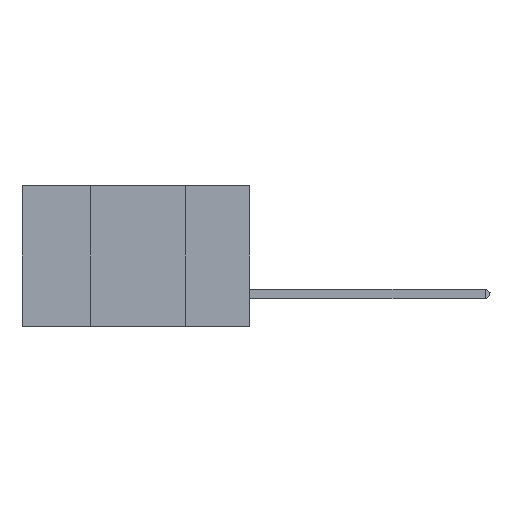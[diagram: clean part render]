
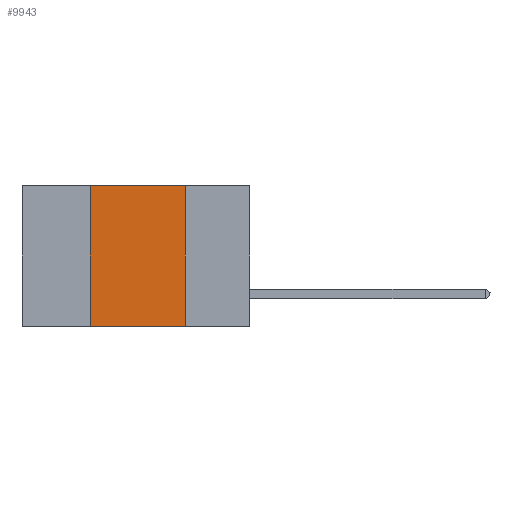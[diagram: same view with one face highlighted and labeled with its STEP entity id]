
A CAD part, left-side view. The second image highlights one B-rep face of the part: STEP entity #9943.
In plain terms, the highlighted planar face has unit normal (-1, 0, 0).
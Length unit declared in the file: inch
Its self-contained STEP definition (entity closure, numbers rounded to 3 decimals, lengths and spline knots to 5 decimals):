
#1324 = DIRECTION ( 'NONE',  ( 0., 0., -1. ) ) ;
#1673 = VERTEX_POINT ( 'NONE', #23737 ) ;
#1791 = VERTEX_POINT ( 'NONE', #7109 ) ;
#2474 = CARTESIAN_POINT ( 'NONE',  ( 0., 0.6, -0.37 ) ) ;
#3134 = EDGE_LOOP ( 'NONE', ( #27689, #11336, #5926, #3174 ) ) ;
#3174 = ORIENTED_EDGE ( 'NONE', *, *, #14783, .T. ) ;
#4747 = DIRECTION ( 'NONE',  ( 0., -1., 0. ) ) ;
#4845 = VERTEX_POINT ( 'NONE', #7659 ) ;
#5437 = LINE ( 'NONE', #11304, #21338 ) ;
#5926 = ORIENTED_EDGE ( 'NONE', *, *, #7079, .F. ) ;
#7079 = EDGE_CURVE ( 'NONE', #1791, #1673, #15362, .T. ) ;
#7109 = CARTESIAN_POINT ( 'NONE',  ( 0., 0.42, -0.37 ) ) ;
#7474 = CARTESIAN_POINT ( 'NONE',  ( 0., 0.17, 0. ) ) ;
#7659 = CARTESIAN_POINT ( 'NONE',  ( 0., 0.17, 0. ) ) ;
#7998 = DIRECTION ( 'NONE',  ( 0., 0., 1. ) ) ;
#8014 = AXIS2_PLACEMENT_3D ( 'NONE', #25604, #8137, #12645 ) ;
#8137 = DIRECTION ( 'NONE',  ( 1., 0., 0. ) ) ;
#8417 = PLANE ( 'NONE',  #8014 ) ;
#8836 = FACE_OUTER_BOUND ( 'NONE', #3134, .T. ) ;
#8990 = VERTEX_POINT ( 'NONE', #17255 ) ;
#9943 = ADVANCED_FACE ( 'NONE', ( #8836 ), #8417, .F. ) ;
#10799 = EDGE_CURVE ( 'NONE', #4845, #8990, #26341, .T. ) ;
#11304 = CARTESIAN_POINT ( 'NONE',  ( 0., 0.6, 0. ) ) ;
#11336 = ORIENTED_EDGE ( 'NONE', *, *, #21173, .F. ) ;
#12645 = DIRECTION ( 'NONE',  ( 0., 0., -1. ) ) ;
#13061 = DIRECTION ( 'NONE',  ( 0., -1., 0. ) ) ;
#14483 = CARTESIAN_POINT ( 'NONE',  ( 0., 0.42, 0. ) ) ;
#14783 = EDGE_CURVE ( 'NONE', #1791, #8990, #19414, .T. ) ;
#15362 = LINE ( 'NONE', #14483, #20505 ) ;
#17255 = CARTESIAN_POINT ( 'NONE',  ( 0., 0.17, -0.37 ) ) ;
#17872 = VECTOR ( 'NONE', #1324, 39.37008 ) ;
#19414 = LINE ( 'NONE', #2474, #20068 ) ;
#20068 = VECTOR ( 'NONE', #4747, 39.37008 ) ;
#20505 = VECTOR ( 'NONE', #7998, 39.37008 ) ;
#21173 = EDGE_CURVE ( 'NONE', #1673, #4845, #5437, .T. ) ;
#21338 = VECTOR ( 'NONE', #13061, 39.37008 ) ;
#23737 = CARTESIAN_POINT ( 'NONE',  ( 0., 0.42, 0. ) ) ;
#25604 = CARTESIAN_POINT ( 'NONE',  ( 0., 0.6, 0. ) ) ;
#26341 = LINE ( 'NONE', #7474, #17872 ) ;
#27689 = ORIENTED_EDGE ( 'NONE', *, *, #10799, .F. ) ;
